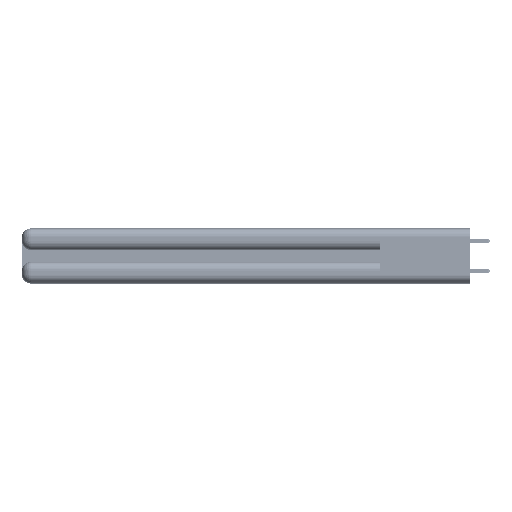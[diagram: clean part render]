
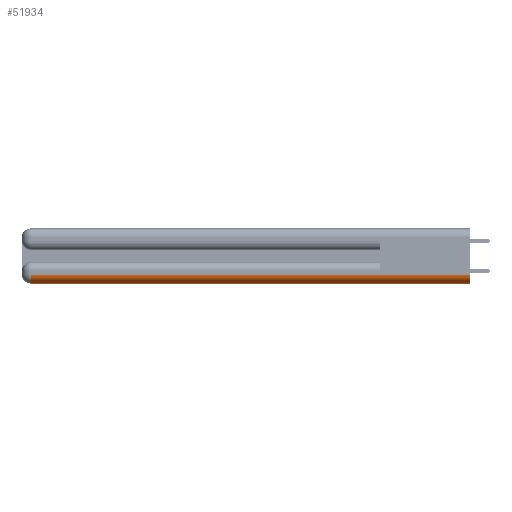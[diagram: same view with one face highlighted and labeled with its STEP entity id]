
A CAD part, left-side view. The second image highlights one B-rep face of the part: STEP entity #51934.
In plain terms, the highlighted cylindrical face has radius 1.524 mm (diameter 3.048 mm), a partial arc.
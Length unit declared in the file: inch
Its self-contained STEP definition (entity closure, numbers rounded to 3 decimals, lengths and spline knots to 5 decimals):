
#1795 = VERTEX_POINT ( 'NONE', #11332 ) ;
#2728 = ORIENTED_EDGE ( 'NONE', *, *, #18873, .F. ) ;
#3365 = DIRECTION ( 'NONE',  ( 0., 1., 0. ) ) ;
#5425 = DIRECTION ( 'NONE',  ( 0., 1., 0. ) ) ;
#9500 = CARTESIAN_POINT ( 'NONE',  ( 0.06, 2.94, 0.06 ) ) ;
#9798 = LINE ( 'NONE', #21238, #25807 ) ;
#11332 = CARTESIAN_POINT ( 'NONE',  ( 0.06, 0., 0. ) ) ;
#12884 = CARTESIAN_POINT ( 'NONE',  ( 0.06, 0., 0.06 ) ) ;
#13541 = CARTESIAN_POINT ( 'NONE',  ( 0.06, 0., 0.06 ) ) ;
#13959 = DIRECTION ( 'NONE',  ( 0., 1., 0. ) ) ;
#16292 = FACE_OUTER_BOUND ( 'NONE', #50443, .T. ) ;
#16577 = DIRECTION ( 'NONE',  ( 0., -1., 0. ) ) ;
#17990 = EDGE_CURVE ( 'NONE', #37764, #32172, #9798, .T. ) ;
#18873 = EDGE_CURVE ( 'NONE', #51150, #37764, #38879, .T. ) ;
#21238 = CARTESIAN_POINT ( 'NONE',  ( 0., 0., 0.06 ) ) ;
#24146 = ORIENTED_EDGE ( 'NONE', *, *, #17990, .F. ) ;
#25730 = DIRECTION ( 'NONE',  ( 0., 0., 1. ) ) ;
#25807 = VECTOR ( 'NONE', #16577, 39.37008 ) ;
#27187 = DIRECTION ( 'NONE',  ( 0., 0., 1. ) ) ;
#27997 = VECTOR ( 'NONE', #5425, 39.37008 ) ;
#28971 = CIRCLE ( 'NONE', #35519, 0.06 ) ;
#29525 = CARTESIAN_POINT ( 'NONE',  ( 0., 2.94, 0.06 ) ) ;
#32172 = VERTEX_POINT ( 'NONE', #32820 ) ;
#32793 = EDGE_CURVE ( 'NONE', #32172, #1795, #28971, .T. ) ;
#32820 = CARTESIAN_POINT ( 'NONE',  ( 0., 0., 0.06 ) ) ;
#33158 = ORIENTED_EDGE ( 'NONE', *, *, #32793, .F. ) ;
#33160 = CARTESIAN_POINT ( 'NONE',  ( 0.06, 2.94, 0. ) ) ;
#33651 = AXIS2_PLACEMENT_3D ( 'NONE', #12884, #3365, #25730 ) ;
#35519 = AXIS2_PLACEMENT_3D ( 'NONE', #13541, #40010, #35908 ) ;
#35706 = EDGE_CURVE ( 'NONE', #1795, #51150, #48919, .T. ) ;
#35908 = DIRECTION ( 'NONE',  ( 0., 0., 1. ) ) ;
#36749 = CARTESIAN_POINT ( 'NONE',  ( 0.06, 3., 0. ) ) ;
#37764 = VERTEX_POINT ( 'NONE', #29525 ) ;
#38879 = CIRCLE ( 'NONE', #57105, 0.06 ) ;
#40010 = DIRECTION ( 'NONE',  ( 0., -1., 0. ) ) ;
#42765 = CYLINDRICAL_SURFACE ( 'NONE', #33651, 0.06 ) ;
#48919 = LINE ( 'NONE', #36749, #27997 ) ;
#50443 = EDGE_LOOP ( 'NONE', ( #33158, #24146, #2728, #53988 ) ) ;
#51150 = VERTEX_POINT ( 'NONE', #33160 ) ;
#51934 = ADVANCED_FACE ( 'NONE', ( #16292 ), #42765, .T. ) ;
#53988 = ORIENTED_EDGE ( 'NONE', *, *, #35706, .F. ) ;
#57105 = AXIS2_PLACEMENT_3D ( 'NONE', #9500, #13959, #27187 ) ;
